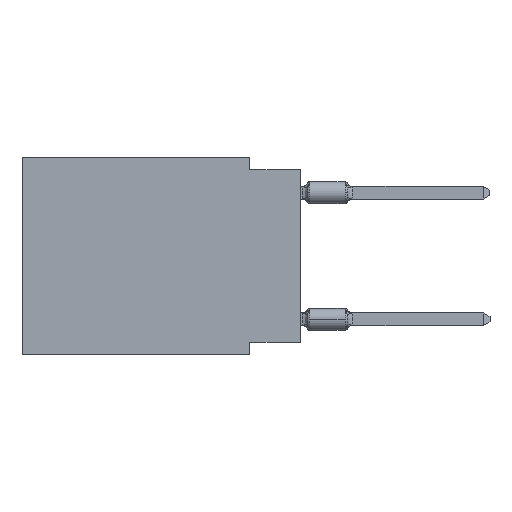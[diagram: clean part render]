
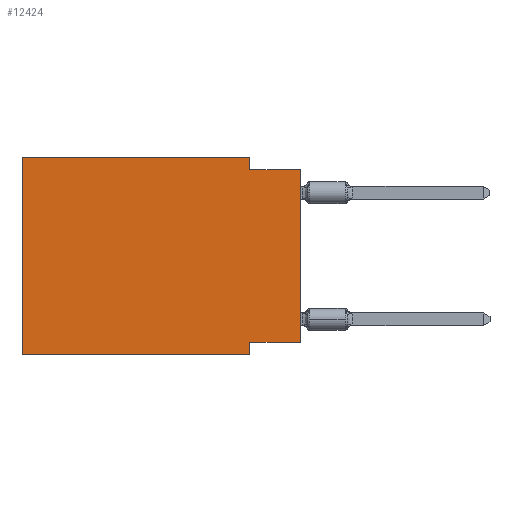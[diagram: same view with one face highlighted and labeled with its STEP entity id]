
A CAD part, left-side view. The second image highlights one B-rep face of the part: STEP entity #12424.
In plain terms, the highlighted planar face has unit normal (-1, 0, 0).
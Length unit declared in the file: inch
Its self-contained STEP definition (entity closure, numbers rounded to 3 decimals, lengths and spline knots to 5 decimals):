
#100 = FACE_OUTER_BOUND ( 'NONE', #7831, .T. ) ;
#211 = EDGE_CURVE ( 'NONE', #11890, #4157, #16194, .T. ) ;
#215 = PLANE ( 'NONE',  #9812 ) ;
#387 = ORIENTED_EDGE ( 'NONE', *, *, #4413, .F. ) ;
#932 = VERTEX_POINT ( 'NONE', #15868 ) ;
#1065 = EDGE_CURVE ( 'NONE', #18577, #19152, #7376, .T. ) ;
#1294 = LINE ( 'NONE', #11819, #18230 ) ;
#1793 = CARTESIAN_POINT ( 'NONE',  ( 0., 0.55, -0.39 ) ) ;
#2232 = DIRECTION ( 'NONE',  ( 0., -1., 0. ) ) ;
#2653 = CARTESIAN_POINT ( 'NONE',  ( 0., 0., -0.365 ) ) ;
#2791 = ORIENTED_EDGE ( 'NONE', *, *, #19983, .T. ) ;
#2816 = EDGE_CURVE ( 'NONE', #19152, #11890, #8258, .T. ) ;
#3859 = CARTESIAN_POINT ( 'NONE',  ( 0., 0., -0.025 ) ) ;
#4157 = VERTEX_POINT ( 'NONE', #3859 ) ;
#4413 = EDGE_CURVE ( 'NONE', #14542, #18577, #20896, .T. ) ;
#5671 = DIRECTION ( 'NONE',  ( 0., -1., 0. ) ) ;
#6281 = LINE ( 'NONE', #16743, #18925 ) ;
#7376 = LINE ( 'NONE', #14388, #16109 ) ;
#7545 = ORIENTED_EDGE ( 'NONE', *, *, #11291, .F. ) ;
#7760 = LINE ( 'NONE', #2653, #10136 ) ;
#7831 = EDGE_LOOP ( 'NONE', ( #20267, #16518, #22334, #10432, #387, #2791, #10645, #7545 ) ) ;
#8258 = LINE ( 'NONE', #15028, #13896 ) ;
#9159 = CARTESIAN_POINT ( 'NONE',  ( 0., 0.55, -0.39 ) ) ;
#9204 = VECTOR ( 'NONE', #5671, 39.37008 ) ;
#9350 = CARTESIAN_POINT ( 'NONE',  ( 0., 0., -0.365 ) ) ;
#9499 = VERTEX_POINT ( 'NONE', #15253 ) ;
#9567 = DIRECTION ( 'NONE',  ( 0., -1., 0. ) ) ;
#9812 = AXIS2_PLACEMENT_3D ( 'NONE', #12459, #10396, #10739 ) ;
#9872 = DIRECTION ( 'NONE',  ( 0., 0., 1. ) ) ;
#10136 = VECTOR ( 'NONE', #19844, 39.37008 ) ;
#10396 = DIRECTION ( 'NONE',  ( 1., 0., 0. ) ) ;
#10432 = ORIENTED_EDGE ( 'NONE', *, *, #1065, .F. ) ;
#10645 = ORIENTED_EDGE ( 'NONE', *, *, #10844, .F. ) ;
#10739 = DIRECTION ( 'NONE',  ( 0., 0., -1. ) ) ;
#10844 = EDGE_CURVE ( 'NONE', #932, #9499, #6281, .T. ) ;
#10870 = LINE ( 'NONE', #9159, #9204 ) ;
#11027 = CARTESIAN_POINT ( 'NONE',  ( 0., 0., -0.025 ) ) ;
#11291 = EDGE_CURVE ( 'NONE', #17776, #932, #7760, .T. ) ;
#11785 = EDGE_CURVE ( 'NONE', #17776, #4157, #1294, .T. ) ;
#11819 = CARTESIAN_POINT ( 'NONE',  ( 0., 0., 0. ) ) ;
#11890 = VERTEX_POINT ( 'NONE', #13882 ) ;
#12424 = ADVANCED_FACE ( 'NONE', ( #100 ), #215, .F. ) ;
#12459 = CARTESIAN_POINT ( 'NONE',  ( 0., 0.55, 0. ) ) ;
#13882 = CARTESIAN_POINT ( 'NONE',  ( 0., 0.1, -0.025 ) ) ;
#13896 = VECTOR ( 'NONE', #16654, 39.37008 ) ;
#14388 = CARTESIAN_POINT ( 'NONE',  ( 0., 0.55, 0. ) ) ;
#14542 = VERTEX_POINT ( 'NONE', #1793 ) ;
#14894 = DIRECTION ( 'NONE',  ( 0., 0., -1. ) ) ;
#15028 = CARTESIAN_POINT ( 'NONE',  ( 0., 0.1, 0. ) ) ;
#15253 = CARTESIAN_POINT ( 'NONE',  ( 0., 0.1, -0.39 ) ) ;
#15868 = CARTESIAN_POINT ( 'NONE',  ( 0., 0.1, -0.365 ) ) ;
#16109 = VECTOR ( 'NONE', #9567, 39.37008 ) ;
#16125 = CARTESIAN_POINT ( 'NONE',  ( 0., 0.1, 0. ) ) ;
#16194 = LINE ( 'NONE', #11027, #17265 ) ;
#16518 = ORIENTED_EDGE ( 'NONE', *, *, #211, .F. ) ;
#16654 = DIRECTION ( 'NONE',  ( 0., 0., -1. ) ) ;
#16743 = CARTESIAN_POINT ( 'NONE',  ( 0., 0.1, -0.39 ) ) ;
#17127 = VECTOR ( 'NONE', #22599, 39.37008 ) ;
#17265 = VECTOR ( 'NONE', #2232, 39.37008 ) ;
#17776 = VERTEX_POINT ( 'NONE', #9350 ) ;
#18230 = VECTOR ( 'NONE', #9872, 39.37008 ) ;
#18577 = VERTEX_POINT ( 'NONE', #19267 ) ;
#18925 = VECTOR ( 'NONE', #14894, 39.37008 ) ;
#19152 = VERTEX_POINT ( 'NONE', #16125 ) ;
#19267 = CARTESIAN_POINT ( 'NONE',  ( 0., 0.55, 0. ) ) ;
#19276 = CARTESIAN_POINT ( 'NONE',  ( 0., 0.55, 0. ) ) ;
#19844 = DIRECTION ( 'NONE',  ( 0., 1., 0. ) ) ;
#19983 = EDGE_CURVE ( 'NONE', #14542, #9499, #10870, .T. ) ;
#20267 = ORIENTED_EDGE ( 'NONE', *, *, #11785, .T. ) ;
#20896 = LINE ( 'NONE', #19276, #17127 ) ;
#22334 = ORIENTED_EDGE ( 'NONE', *, *, #2816, .F. ) ;
#22599 = DIRECTION ( 'NONE',  ( 0., 0., 1. ) ) ;
